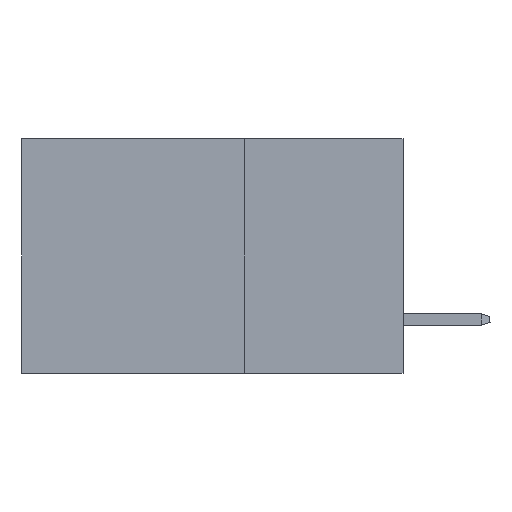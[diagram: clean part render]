
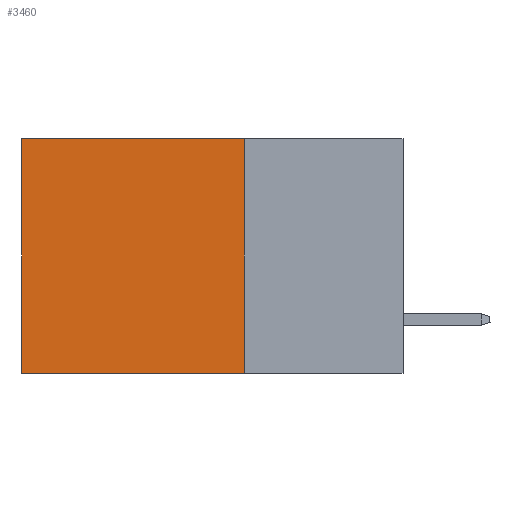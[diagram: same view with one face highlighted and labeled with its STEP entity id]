
A CAD part, left-side view. The second image highlights one B-rep face of the part: STEP entity #3460.
In plain terms, the highlighted planar face has unit normal (-1, 0, 0).
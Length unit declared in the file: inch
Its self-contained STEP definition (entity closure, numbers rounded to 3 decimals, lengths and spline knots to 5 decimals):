
#2496 = ORIENTED_EDGE ( 'NONE', *, *, #17961, .T. ) ;
#3460 = ADVANCED_FACE ( 'NONE', ( #23203 ), #17284, .F. ) ;
#7791 = CARTESIAN_POINT ( 'NONE',  ( 0.2875, 0.6, 0. ) ) ;
#10433 = LINE ( 'NONE', #11670, #11123 ) ;
#10470 = LINE ( 'NONE', #7791, #25678 ) ;
#10660 = EDGE_LOOP ( 'NONE', ( #2496, #24258, #29062, #15198 ) ) ;
#10911 = EDGE_CURVE ( 'NONE', #18532, #11449, #29789, .T. ) ;
#11123 = VECTOR ( 'NONE', #27780, 39.37008 ) ;
#11386 = EDGE_CURVE ( 'NONE', #18532, #25270, #10433, .T. ) ;
#11449 = VERTEX_POINT ( 'NONE', #11484 ) ;
#11484 = CARTESIAN_POINT ( 'NONE',  ( 0.2875, 0.6, 0. ) ) ;
#11670 = CARTESIAN_POINT ( 'NONE',  ( 0.2875, 0.25, 0. ) ) ;
#12856 = VECTOR ( 'NONE', #27110, 39.37008 ) ;
#14591 = CARTESIAN_POINT ( 'NONE',  ( 0.2875, 0.25, -0.37 ) ) ;
#14974 = CARTESIAN_POINT ( 'NONE',  ( 0.2875, 0.25, 0. ) ) ;
#15198 = ORIENTED_EDGE ( 'NONE', *, *, #10911, .T. ) ;
#15289 = AXIS2_PLACEMENT_3D ( 'NONE', #14974, #28213, #20161 ) ;
#16007 = DIRECTION ( 'NONE',  ( 0., 0., -1. ) ) ;
#17284 = PLANE ( 'NONE',  #15289 ) ;
#17961 = EDGE_CURVE ( 'NONE', #11449, #18807, #10470, .T. ) ;
#18532 = VERTEX_POINT ( 'NONE', #35192 ) ;
#18807 = VERTEX_POINT ( 'NONE', #24760 ) ;
#20161 = DIRECTION ( 'NONE',  ( 0., 0., -1. ) ) ;
#20318 = LINE ( 'NONE', #14591, #34999 ) ;
#23190 = DIRECTION ( 'NONE',  ( 0., 1., 0. ) ) ;
#23203 = FACE_OUTER_BOUND ( 'NONE', #10660, .T. ) ;
#24258 = ORIENTED_EDGE ( 'NONE', *, *, #31657, .F. ) ;
#24760 = CARTESIAN_POINT ( 'NONE',  ( 0.2875, 0.6, -0.37 ) ) ;
#25270 = VERTEX_POINT ( 'NONE', #35111 ) ;
#25678 = VECTOR ( 'NONE', #16007, 39.37008 ) ;
#26935 = CARTESIAN_POINT ( 'NONE',  ( 0.2875, 0.25, 0. ) ) ;
#27110 = DIRECTION ( 'NONE',  ( 0., 1., 0. ) ) ;
#27780 = DIRECTION ( 'NONE',  ( 0., 0., -1. ) ) ;
#28213 = DIRECTION ( 'NONE',  ( 1., 0., 0. ) ) ;
#29062 = ORIENTED_EDGE ( 'NONE', *, *, #11386, .F. ) ;
#29789 = LINE ( 'NONE', #26935, #12856 ) ;
#31657 = EDGE_CURVE ( 'NONE', #25270, #18807, #20318, .T. ) ;
#34999 = VECTOR ( 'NONE', #23190, 39.37008 ) ;
#35111 = CARTESIAN_POINT ( 'NONE',  ( 0.2875, 0.25, -0.37 ) ) ;
#35192 = CARTESIAN_POINT ( 'NONE',  ( 0.2875, 0.25, 0. ) ) ;
